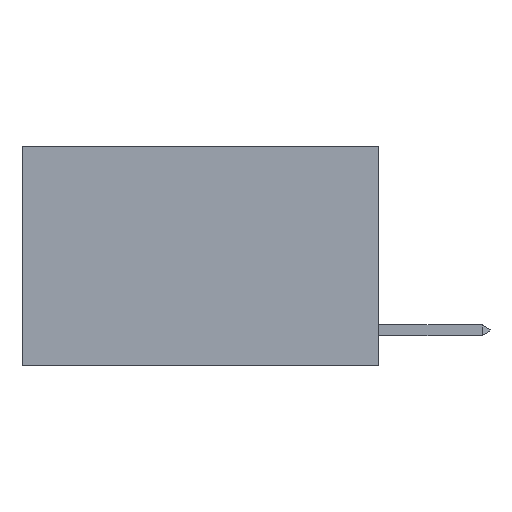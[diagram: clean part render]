
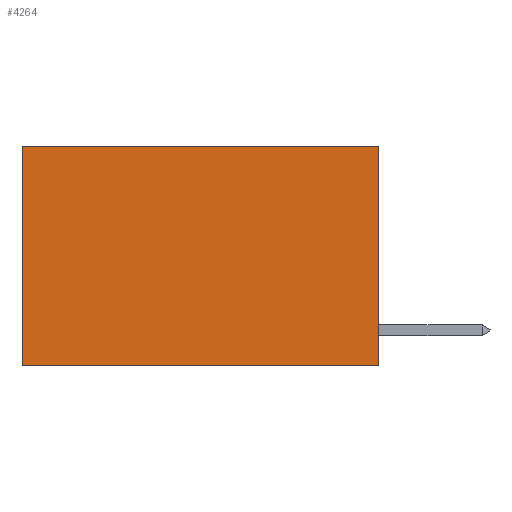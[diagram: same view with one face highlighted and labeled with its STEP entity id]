
A CAD part, left-side view. The second image highlights one B-rep face of the part: STEP entity #4264.
In plain terms, the highlighted planar face has unit normal (-1, 0, 0).
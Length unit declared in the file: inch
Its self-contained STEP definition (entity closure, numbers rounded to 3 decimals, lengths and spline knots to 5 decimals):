
#30 = CARTESIAN_POINT ( 'NONE',  ( 0.2625, 0., 0. ) ) ;
#487 = PLANE ( 'NONE',  #1603 ) ;
#715 = VERTEX_POINT ( 'NONE', #2830 ) ;
#1603 = AXIS2_PLACEMENT_3D ( 'NONE', #9399, #3602, #15407 ) ;
#2141 = CARTESIAN_POINT ( 'NONE',  ( 0.2625, 0., -0.37 ) ) ;
#2232 = EDGE_CURVE ( 'NONE', #15359, #715, #10166, .T. ) ;
#2830 = CARTESIAN_POINT ( 'NONE',  ( 0.2625, 0.6, 0. ) ) ;
#3461 = CARTESIAN_POINT ( 'NONE',  ( 0.2625, 0.6, 0. ) ) ;
#3602 = DIRECTION ( 'NONE',  ( 1., 0., 0. ) ) ;
#4264 = ADVANCED_FACE ( 'NONE', ( #5544 ), #487, .F. ) ;
#4535 = VECTOR ( 'NONE', #4899, 39.37008 ) ;
#4623 = CARTESIAN_POINT ( 'NONE',  ( 0.2625, 0.6, -0.37 ) ) ;
#4730 = VECTOR ( 'NONE', #10885, 39.37008 ) ;
#4899 = DIRECTION ( 'NONE',  ( 0., 0., -1. ) ) ;
#5544 = FACE_OUTER_BOUND ( 'NONE', #9758, .T. ) ;
#6860 = DIRECTION ( 'NONE',  ( 0., 1., 0. ) ) ;
#7101 = ORIENTED_EDGE ( 'NONE', *, *, #16661, .T. ) ;
#7399 = CARTESIAN_POINT ( 'NONE',  ( 0.2625, 0., -0.37 ) ) ;
#8778 = VECTOR ( 'NONE', #6860, 39.37008 ) ;
#8895 = LINE ( 'NONE', #30, #14236 ) ;
#9373 = LINE ( 'NONE', #3461, #4535 ) ;
#9382 = VERTEX_POINT ( 'NONE', #7399 ) ;
#9399 = CARTESIAN_POINT ( 'NONE',  ( 0.2625, 0., 0. ) ) ;
#9758 = EDGE_LOOP ( 'NONE', ( #7101, #15874, #17431, #12715 ) ) ;
#10166 = LINE ( 'NONE', #18649, #8778 ) ;
#10375 = DIRECTION ( 'NONE',  ( 0., 0., -1. ) ) ;
#10431 = VERTEX_POINT ( 'NONE', #4623 ) ;
#10885 = DIRECTION ( 'NONE',  ( 0., 1., 0. ) ) ;
#12715 = ORIENTED_EDGE ( 'NONE', *, *, #2232, .T. ) ;
#13742 = LINE ( 'NONE', #2141, #4730 ) ;
#14217 = CARTESIAN_POINT ( 'NONE',  ( 0.2625, 0., 0. ) ) ;
#14236 = VECTOR ( 'NONE', #10375, 39.37008 ) ;
#15359 = VERTEX_POINT ( 'NONE', #14217 ) ;
#15407 = DIRECTION ( 'NONE',  ( 0., 0., -1. ) ) ;
#15874 = ORIENTED_EDGE ( 'NONE', *, *, #17297, .F. ) ;
#16661 = EDGE_CURVE ( 'NONE', #715, #10431, #9373, .T. ) ;
#17076 = EDGE_CURVE ( 'NONE', #15359, #9382, #8895, .T. ) ;
#17297 = EDGE_CURVE ( 'NONE', #9382, #10431, #13742, .T. ) ;
#17431 = ORIENTED_EDGE ( 'NONE', *, *, #17076, .F. ) ;
#18649 = CARTESIAN_POINT ( 'NONE',  ( 0.2625, 0., 0. ) ) ;
